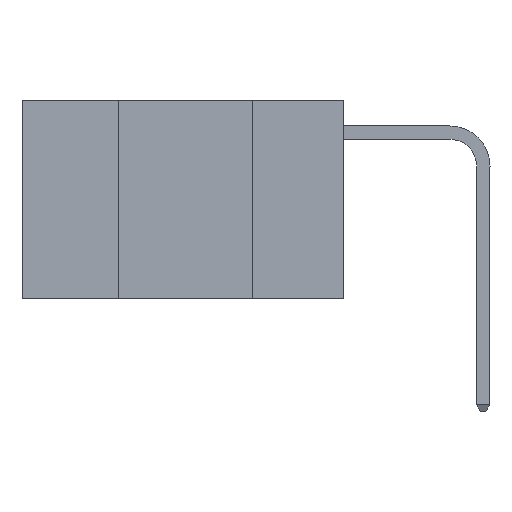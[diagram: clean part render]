
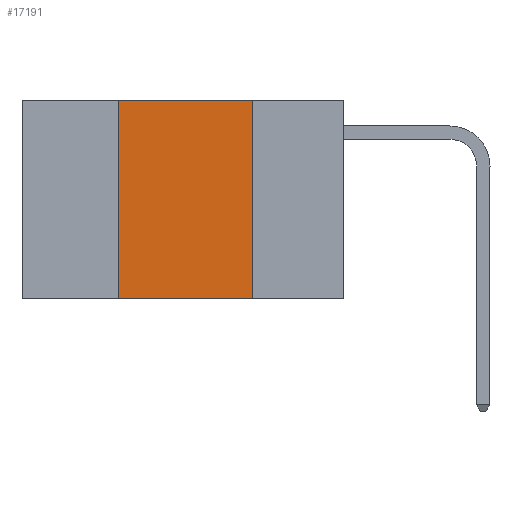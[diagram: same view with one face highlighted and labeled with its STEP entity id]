
A CAD part, left-side view. The second image highlights one B-rep face of the part: STEP entity #17191.
In plain terms, the highlighted planar face has unit normal (-1, 0, 0).
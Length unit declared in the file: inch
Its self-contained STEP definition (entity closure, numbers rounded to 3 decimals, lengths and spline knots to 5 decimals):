
#396 = EDGE_LOOP ( 'NONE', ( #15599, #12538, #11387, #10336 ) ) ;
#980 = PLANE ( 'NONE',  #2368 ) ;
#1880 = CARTESIAN_POINT ( 'NONE',  ( 0., 0.17, 0. ) ) ;
#2368 = AXIS2_PLACEMENT_3D ( 'NONE', #2454, #11797, #3806 ) ;
#2454 = CARTESIAN_POINT ( 'NONE',  ( 0., 0.6, 0. ) ) ;
#2990 = VERTEX_POINT ( 'NONE', #7801 ) ;
#3161 = FACE_OUTER_BOUND ( 'NONE', #396, .T. ) ;
#3369 = LINE ( 'NONE', #15584, #17188 ) ;
#3667 = CARTESIAN_POINT ( 'NONE',  ( 0., 0.42, -0.37 ) ) ;
#3806 = DIRECTION ( 'NONE',  ( 0., 0., -1. ) ) ;
#4102 = VECTOR ( 'NONE', #5354, 39.37008 ) ;
#4559 = EDGE_CURVE ( 'NONE', #15034, #16387, #3369, .T. ) ;
#5354 = DIRECTION ( 'NONE',  ( 0., -1., 0. ) ) ;
#5546 = EDGE_CURVE ( 'NONE', #8037, #16387, #6094, .T. ) ;
#6094 = LINE ( 'NONE', #16200, #12314 ) ;
#7566 = CARTESIAN_POINT ( 'NONE',  ( 0., 0.17, -0.37 ) ) ;
#7602 = EDGE_CURVE ( 'NONE', #2990, #15034, #13912, .T. ) ;
#7801 = CARTESIAN_POINT ( 'NONE',  ( 0., 0.42, 0. ) ) ;
#8037 = VERTEX_POINT ( 'NONE', #3667 ) ;
#10103 = LINE ( 'NONE', #12417, #16774 ) ;
#10336 = ORIENTED_EDGE ( 'NONE', *, *, #5546, .T. ) ;
#10689 = CARTESIAN_POINT ( 'NONE',  ( 0., 0.6, 0. ) ) ;
#11387 = ORIENTED_EDGE ( 'NONE', *, *, #14418, .F. ) ;
#11797 = DIRECTION ( 'NONE',  ( 1., 0., 0. ) ) ;
#12314 = VECTOR ( 'NONE', #14913, 39.37008 ) ;
#12417 = CARTESIAN_POINT ( 'NONE',  ( 0., 0.42, 0. ) ) ;
#12538 = ORIENTED_EDGE ( 'NONE', *, *, #7602, .F. ) ;
#13759 = DIRECTION ( 'NONE',  ( 0., 0., 1. ) ) ;
#13912 = LINE ( 'NONE', #10689, #4102 ) ;
#14418 = EDGE_CURVE ( 'NONE', #8037, #2990, #10103, .T. ) ;
#14913 = DIRECTION ( 'NONE',  ( 0., -1., 0. ) ) ;
#15034 = VERTEX_POINT ( 'NONE', #1880 ) ;
#15584 = CARTESIAN_POINT ( 'NONE',  ( 0., 0.17, 0. ) ) ;
#15599 = ORIENTED_EDGE ( 'NONE', *, *, #4559, .F. ) ;
#16200 = CARTESIAN_POINT ( 'NONE',  ( 0., 0.6, -0.37 ) ) ;
#16387 = VERTEX_POINT ( 'NONE', #7566 ) ;
#16774 = VECTOR ( 'NONE', #13759, 39.37008 ) ;
#16917 = DIRECTION ( 'NONE',  ( 0., 0., -1. ) ) ;
#17188 = VECTOR ( 'NONE', #16917, 39.37008 ) ;
#17191 = ADVANCED_FACE ( 'NONE', ( #3161 ), #980, .F. ) ;
